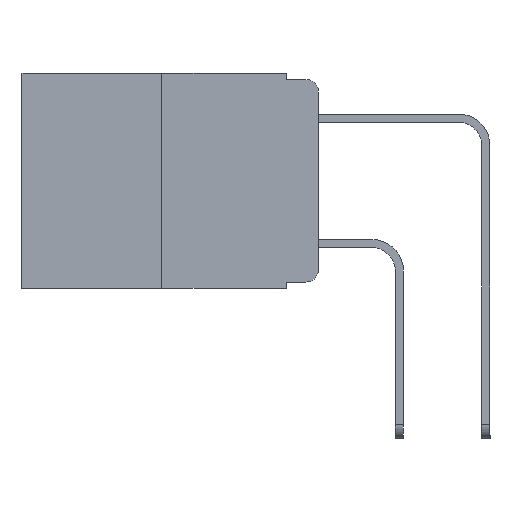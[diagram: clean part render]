
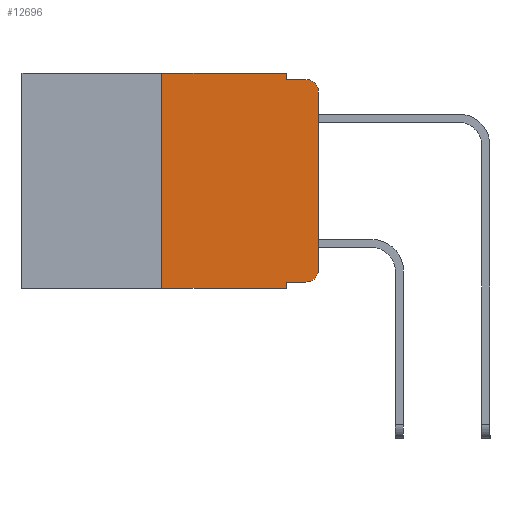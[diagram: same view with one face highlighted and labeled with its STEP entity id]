
A CAD part, left-side view. The second image highlights one B-rep face of the part: STEP entity #12696.
In plain terms, the highlighted planar face has unit normal (-1, 0, 0).
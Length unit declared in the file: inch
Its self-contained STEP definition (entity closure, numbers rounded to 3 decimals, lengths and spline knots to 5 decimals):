
#1627 = VERTEX_POINT ( 'NONE', #20047 ) ;
#1961 = DIRECTION ( 'NONE',  ( 0., -1., 0. ) ) ;
#2141 = VERTEX_POINT ( 'NONE', #10664 ) ;
#2426 = CARTESIAN_POINT ( 'NONE',  ( 0., 0.473, -0.343 ) ) ;
#2821 = VECTOR ( 'NONE', #6987, 39.37008 ) ;
#3212 = EDGE_CURVE ( 'NONE', #1627, #25276, #10402, .T. ) ;
#3471 = DIRECTION ( 'NONE',  ( 0., -1., 0. ) ) ;
#3789 = CARTESIAN_POINT ( 'NONE',  ( 0., 0.051, 0. ) ) ;
#3881 = CARTESIAN_POINT ( 'NONE',  ( 0., 0.051, 0. ) ) ;
#4101 = LINE ( 'NONE', #11103, #2821 ) ;
#4528 = ORIENTED_EDGE ( 'NONE', *, *, #19440, .F. ) ;
#4545 = EDGE_CURVE ( 'NONE', #1627, #2141, #21968, .T. ) ;
#4750 = CARTESIAN_POINT ( 'NONE',  ( 0., 0.02, -0.313 ) ) ;
#4884 = CARTESIAN_POINT ( 'NONE',  ( 0., 0.051, -0.01 ) ) ;
#5395 = PLANE ( 'NONE',  #22177 ) ;
#5432 = LINE ( 'NONE', #21644, #20276 ) ;
#5827 = VERTEX_POINT ( 'NONE', #21706 ) ;
#5931 = EDGE_CURVE ( 'NONE', #13968, #25276, #6474, .T. ) ;
#6087 = DIRECTION ( 'NONE',  ( 0., -1., 0. ) ) ;
#6200 = EDGE_CURVE ( 'NONE', #8185, #25850, #22451, .T. ) ;
#6474 = LINE ( 'NONE', #3881, #21897 ) ;
#6813 = CARTESIAN_POINT ( 'NONE',  ( 0., 0.473, 0. ) ) ;
#6818 = DIRECTION ( 'NONE',  ( 0., 0., -1. ) ) ;
#6867 = VECTOR ( 'NONE', #18872, 39.37008 ) ;
#6987 = DIRECTION ( 'NONE',  ( 0., 0., 1. ) ) ;
#7054 = ORIENTED_EDGE ( 'NONE', *, *, #8118, .T. ) ;
#7990 = CARTESIAN_POINT ( 'NONE',  ( 0., 0.02, -0.03 ) ) ;
#8118 = EDGE_CURVE ( 'NONE', #25850, #16668, #4101, .T. ) ;
#8185 = VERTEX_POINT ( 'NONE', #17301 ) ;
#8927 = AXIS2_PLACEMENT_3D ( 'NONE', #7990, #22056, #10056 ) ;
#9419 = CIRCLE ( 'NONE', #8927, 0.02 ) ;
#9479 = DIRECTION ( 'NONE',  ( 1., 0., 0. ) ) ;
#10012 = EDGE_CURVE ( 'NONE', #2141, #23090, #17598, .T. ) ;
#10056 = DIRECTION ( 'NONE',  ( 0., 0., -1. ) ) ;
#10402 = LINE ( 'NONE', #2426, #25631 ) ;
#10664 = CARTESIAN_POINT ( 'NONE',  ( 0., 0.25, 0. ) ) ;
#10707 = VERTEX_POINT ( 'NONE', #4884 ) ;
#11103 = CARTESIAN_POINT ( 'NONE',  ( 0., 0., 0. ) ) ;
#11865 = CARTESIAN_POINT ( 'NONE',  ( 0., 0.051, -0.333 ) ) ;
#11978 = VECTOR ( 'NONE', #13214, 39.37008 ) ;
#12696 = ADVANCED_FACE ( 'NONE', ( #15236 ), #5395, .F. ) ;
#12742 = EDGE_CURVE ( 'NONE', #23090, #10707, #24575, .T. ) ;
#12834 = ORIENTED_EDGE ( 'NONE', *, *, #3212, .T. ) ;
#13214 = DIRECTION ( 'NONE',  ( 0., 0., 1. ) ) ;
#13479 = CARTESIAN_POINT ( 'NONE',  ( 0., 0.473, 0. ) ) ;
#13777 = ORIENTED_EDGE ( 'NONE', *, *, #18192, .T. ) ;
#13968 = VERTEX_POINT ( 'NONE', #11865 ) ;
#14020 = DIRECTION ( 'NONE',  ( 0., 0., -1. ) ) ;
#14972 = ORIENTED_EDGE ( 'NONE', *, *, #4545, .F. ) ;
#15236 = FACE_OUTER_BOUND ( 'NONE', #19728, .T. ) ;
#16076 = CARTESIAN_POINT ( 'NONE',  ( 0., 0., -0.03 ) ) ;
#16668 = VERTEX_POINT ( 'NONE', #16076 ) ;
#17301 = CARTESIAN_POINT ( 'NONE',  ( 0., 0.02, -0.333 ) ) ;
#17598 = LINE ( 'NONE', #6813, #6867 ) ;
#17697 = LINE ( 'NONE', #18137, #23617 ) ;
#17811 = CARTESIAN_POINT ( 'NONE',  ( 0., 0.051, -0.343 ) ) ;
#17814 = CARTESIAN_POINT ( 'NONE',  ( 0., 0.25, 0. ) ) ;
#18137 = CARTESIAN_POINT ( 'NONE',  ( 0., 0.051, -0.333 ) ) ;
#18192 = EDGE_CURVE ( 'NONE', #13968, #8185, #17697, .T. ) ;
#18872 = DIRECTION ( 'NONE',  ( 0., -1., 0. ) ) ;
#18884 = DIRECTION ( 'NONE',  ( -1., 0., 0. ) ) ;
#19097 = ORIENTED_EDGE ( 'NONE', *, *, #6200, .T. ) ;
#19337 = VECTOR ( 'NONE', #25513, 39.37008 ) ;
#19440 = EDGE_CURVE ( 'NONE', #10707, #5827, #5432, .T. ) ;
#19728 = EDGE_LOOP ( 'NONE', ( #7054, #23708, #4528, #20635, #24332, #14972, #12834, #23435, #13777, #19097 ) ) ;
#20047 = CARTESIAN_POINT ( 'NONE',  ( 0., 0.25, -0.343 ) ) ;
#20276 = VECTOR ( 'NONE', #3471, 39.37008 ) ;
#20635 = ORIENTED_EDGE ( 'NONE', *, *, #12742, .F. ) ;
#21611 = CARTESIAN_POINT ( 'NONE',  ( 0., 0.051, 0. ) ) ;
#21644 = CARTESIAN_POINT ( 'NONE',  ( 0., 0.051, -0.01 ) ) ;
#21706 = CARTESIAN_POINT ( 'NONE',  ( 0., 0.02, -0.01 ) ) ;
#21897 = VECTOR ( 'NONE', #14020, 39.37008 ) ;
#21968 = LINE ( 'NONE', #17814, #11978 ) ;
#22056 = DIRECTION ( 'NONE',  ( -1., 0., 0. ) ) ;
#22177 = AXIS2_PLACEMENT_3D ( 'NONE', #13479, #9479, #23497 ) ;
#22451 = CIRCLE ( 'NONE', #24238, 0.02 ) ;
#23090 = VERTEX_POINT ( 'NONE', #3789 ) ;
#23435 = ORIENTED_EDGE ( 'NONE', *, *, #5931, .F. ) ;
#23497 = DIRECTION ( 'NONE',  ( 0., 0., -1. ) ) ;
#23617 = VECTOR ( 'NONE', #6087, 39.37008 ) ;
#23708 = ORIENTED_EDGE ( 'NONE', *, *, #25998, .T. ) ;
#24238 = AXIS2_PLACEMENT_3D ( 'NONE', #4750, #18884, #6818 ) ;
#24332 = ORIENTED_EDGE ( 'NONE', *, *, #10012, .F. ) ;
#24575 = LINE ( 'NONE', #21611, #19337 ) ;
#25276 = VERTEX_POINT ( 'NONE', #17811 ) ;
#25366 = CARTESIAN_POINT ( 'NONE',  ( 0., 0., -0.313 ) ) ;
#25513 = DIRECTION ( 'NONE',  ( 0., 0., -1. ) ) ;
#25631 = VECTOR ( 'NONE', #1961, 39.37008 ) ;
#25850 = VERTEX_POINT ( 'NONE', #25366 ) ;
#25998 = EDGE_CURVE ( 'NONE', #16668, #5827, #9419, .T. ) ;
